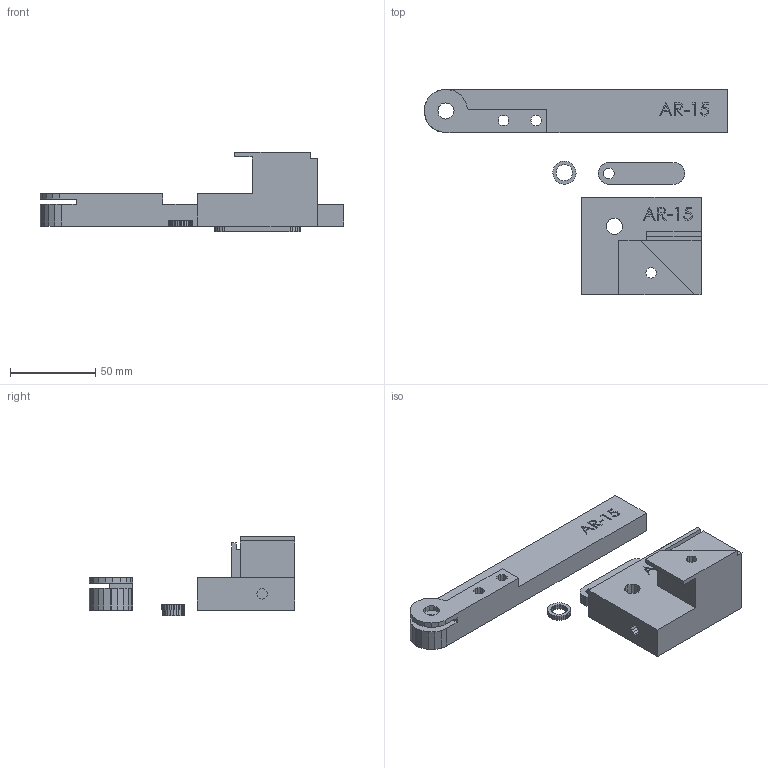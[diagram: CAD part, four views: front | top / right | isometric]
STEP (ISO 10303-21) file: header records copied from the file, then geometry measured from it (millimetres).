
FILE_DESCRIPTION(('STEP AP214'),'1');
FILE_NAME('All parts AR15.stp','2020-03-31T01:17:04',(' '),(' '),'Spatial InterOp 3D',' ',' ');
FILE_SCHEMA(('AUTOMOTIVE_DESIGN { 1 0 10303 214 1 1 1 1 }'));
Length unit declared in the file: metre
Products named in the file (1): Solid
Bounding box: 177.8 x 120.29 x 46.35 mm (x, y, z)
Volume: 167127.9 mm3; surface area: 38424.8 mm2
Topology: 4 solids, 4 shells, 436 faces, 1303 edges, 890 vertices
Faces by surface type: plane 436
Entity records: 14532 total; most frequent: CARTESIAN_POINT 2633, ORIENTED_EDGE 2606, DIRECTION 2183, EDGE_CURVE 1303, LINE 1303, VECTOR 1303, VERTEX_POINT 890, EDGE_LOOP 467
